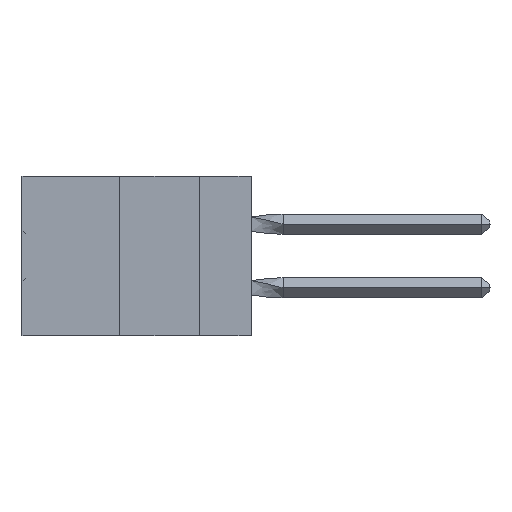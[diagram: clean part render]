
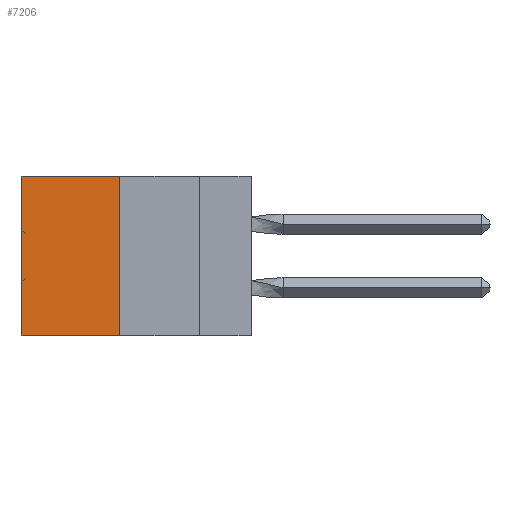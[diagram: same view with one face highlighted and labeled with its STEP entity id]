
A CAD part, left-side view. The second image highlights one B-rep face of the part: STEP entity #7206.
In plain terms, the highlighted planar face has unit normal (-1, 0, 0).
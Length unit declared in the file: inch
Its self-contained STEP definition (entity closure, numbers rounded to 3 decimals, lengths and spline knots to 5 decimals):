
#657 = VERTEX_POINT ( 'NONE', #45734 ) ;
#5526 = CARTESIAN_POINT ( 'NONE',  ( 0.305, 0.72, 0. ) ) ;
#7206 = ADVANCED_FACE ( 'NONE', ( #13226 ), #34768, .F. ) ;
#7381 = VERTEX_POINT ( 'NONE', #5526 ) ;
#7450 = ORIENTED_EDGE ( 'NONE', *, *, #46439, .F. ) ;
#12246 = AXIS2_PLACEMENT_3D ( 'NONE', #17563, #31048, #21844 ) ;
#12323 = CARTESIAN_POINT ( 'NONE',  ( 0.305, 0.413, -0.5 ) ) ;
#13226 = FACE_OUTER_BOUND ( 'NONE', #47010, .T. ) ;
#13523 = LINE ( 'NONE', #23017, #32886 ) ;
#17563 = CARTESIAN_POINT ( 'NONE',  ( 0.305, 0.413, -0.5 ) ) ;
#19385 = EDGE_CURVE ( 'NONE', #7381, #657, #13523, .T. ) ;
#21844 = DIRECTION ( 'NONE',  ( 0., 0., -1. ) ) ;
#22312 = VECTOR ( 'NONE', #31586, 39.37008 ) ;
#22580 = CARTESIAN_POINT ( 'NONE',  ( 0.305, 0.413, -0.5 ) ) ;
#23017 = CARTESIAN_POINT ( 'NONE',  ( 0.305, 0.72, -0.5 ) ) ;
#24915 = ORIENTED_EDGE ( 'NONE', *, *, #36204, .F. ) ;
#26977 = VECTOR ( 'NONE', #54678, 39.37008 ) ;
#27339 = DIRECTION ( 'NONE',  ( 0., 0., -1. ) ) ;
#29802 = VECTOR ( 'NONE', #42255, 39.37008 ) ;
#31048 = DIRECTION ( 'NONE',  ( 1., 0., 0. ) ) ;
#31586 = DIRECTION ( 'NONE',  ( 0., 0., -1. ) ) ;
#32110 = ORIENTED_EDGE ( 'NONE', *, *, #19385, .T. ) ;
#32273 = ORIENTED_EDGE ( 'NONE', *, *, #48376, .T. ) ;
#32886 = VECTOR ( 'NONE', #27339, 39.37008 ) ;
#34768 = PLANE ( 'NONE',  #12246 ) ;
#36204 = EDGE_CURVE ( 'NONE', #40999, #37999, #36378, .T. ) ;
#36378 = LINE ( 'NONE', #22580, #22312 ) ;
#37144 = LINE ( 'NONE', #12323, #29802 ) ;
#37999 = VERTEX_POINT ( 'NONE', #53099 ) ;
#38612 = CARTESIAN_POINT ( 'NONE',  ( 0.305, 0.413, 0. ) ) ;
#40999 = VERTEX_POINT ( 'NONE', #38612 ) ;
#41253 = CARTESIAN_POINT ( 'NONE',  ( 0.305, 0.413, 0. ) ) ;
#42255 = DIRECTION ( 'NONE',  ( 0., 1., 0. ) ) ;
#45734 = CARTESIAN_POINT ( 'NONE',  ( 0.305, 0.72, -0.5 ) ) ;
#46439 = EDGE_CURVE ( 'NONE', #37999, #657, #37144, .T. ) ;
#47010 = EDGE_LOOP ( 'NONE', ( #32110, #7450, #24915, #32273 ) ) ;
#48376 = EDGE_CURVE ( 'NONE', #40999, #7381, #49733, .T. ) ;
#49733 = LINE ( 'NONE', #41253, #26977 ) ;
#53099 = CARTESIAN_POINT ( 'NONE',  ( 0.305, 0.413, -0.5 ) ) ;
#54678 = DIRECTION ( 'NONE',  ( 0., 1., 0. ) ) ;
